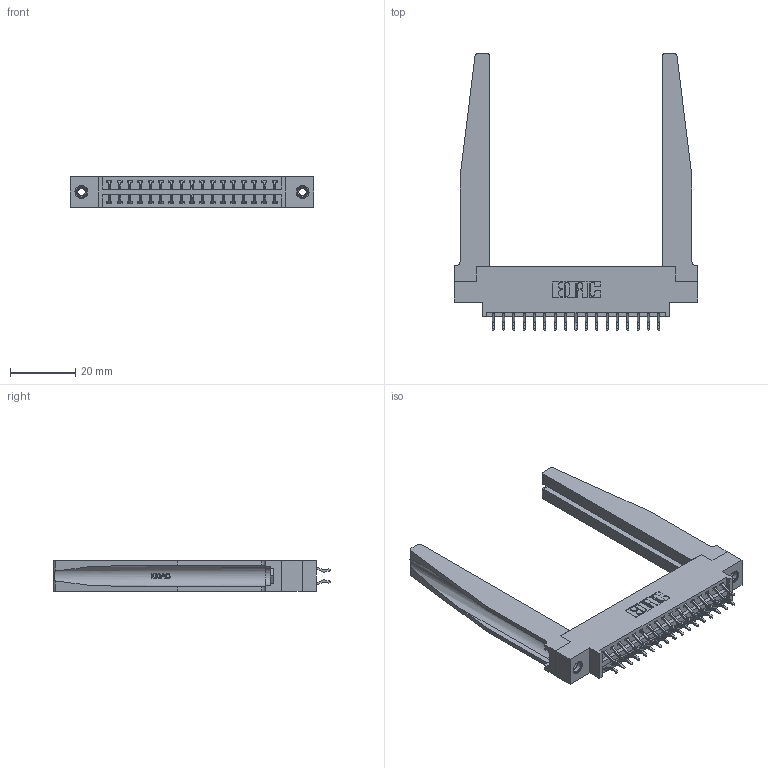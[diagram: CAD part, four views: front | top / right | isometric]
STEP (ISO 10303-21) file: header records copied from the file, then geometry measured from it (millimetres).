
FILE_DESCRIPTION (( 'STEP AP203' ), '1' );
FILE_NAME ('346-034-556-878.STEP', '2022-05-19T20:16:52', ( '' ), ( '' ), 'SwSTEP 2.0', 'SolidWorks 2020', '' );
FILE_SCHEMA (( 'CONFIG_CONTROL_DESIGN' ));
Length unit declared in the file: inch
Products named in the file (5): 346 Part_0.170 Offset - 0.156 Dia-TH; 346-034-556-878; 345-250-001_345-250-001-102; 346-220-078_345-220-078; 345-292-001_556 Tail
Assembly tree (39 placements, depth 2):
  346-034-556-878
    346 Part_0.170 Offset - 0.156 Dia-TH
    345-292-001_556 Tail  x34
    346-220-078_345-220-078  x2
    345-250-001_345-250-001-102  x2
Bounding box: 74.55 x 84.84 x 9.4 mm (x, y, z)
Volume: 13810.1 mm3; surface area: 15813.4 mm2
Topology: 39 solids, 39 shells, 2346 faces, 6867 edges, 4522 vertices
Faces by surface type: plane 1562, cylinder 732, bspline 36, cone 12, torus 4
Entity records: 19976 total; most frequent: CARTESIAN_POINT 4285, ORIENTED_EDGE 3094, DIRECTION 2801, EDGE_CURVE 1547, VECTOR 1245, LINE 1245, VERTEX_POINT 1024, AXIS2_PLACEMENT_3D 778
